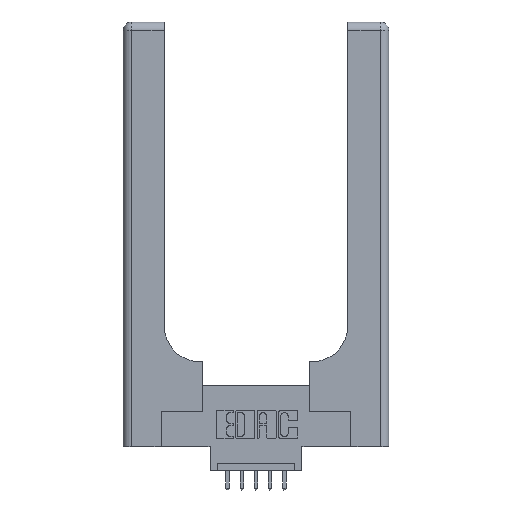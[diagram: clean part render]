
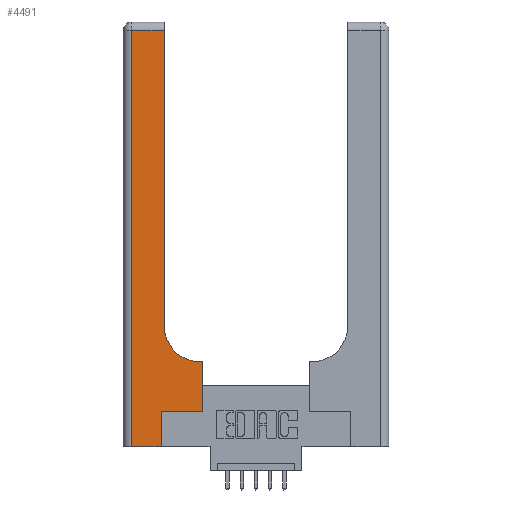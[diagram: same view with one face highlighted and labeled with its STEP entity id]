
A CAD part, top view. The second image highlights one B-rep face of the part: STEP entity #4491.
In plain terms, the highlighted planar face has unit normal (0, 0, 1).
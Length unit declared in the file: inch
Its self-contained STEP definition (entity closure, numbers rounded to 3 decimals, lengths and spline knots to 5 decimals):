
#84 = VERTEX_POINT ( 'NONE', #10954 ) ;
#95 = CARTESIAN_POINT ( 'NONE',  ( 0.5585, 0.6, 0.37 ) ) ;
#163 = CARTESIAN_POINT ( 'NONE',  ( 0., 2.94, 0.37 ) ) ;
#602 = EDGE_CURVE ( 'NONE', #12615, #5786, #12269, .T. ) ;
#630 = VERTEX_POINT ( 'NONE', #1063 ) ;
#729 = CARTESIAN_POINT ( 'NONE',  ( 0.5585, 0.25, 0.37 ) ) ;
#740 = DIRECTION ( 'NONE',  ( -1., 0., 0. ) ) ;
#837 = LINE ( 'NONE', #8546, #9173 ) ;
#874 = LINE ( 'NONE', #163, #2252 ) ;
#981 = EDGE_LOOP ( 'NONE', ( #1285, #3041, #1829, #11075, #13214, #6369, #5208, #11336, #6396 ) ) ;
#1063 = CARTESIAN_POINT ( 'NONE',  ( 0.2915, 2.94, 0.37 ) ) ;
#1086 = EDGE_CURVE ( 'NONE', #630, #84, #874, .T. ) ;
#1156 = LINE ( 'NONE', #11739, #12014 ) ;
#1285 = ORIENTED_EDGE ( 'NONE', *, *, #5250, .T. ) ;
#1527 = CARTESIAN_POINT ( 'NONE',  ( 0.5585, 0.25, 0.37 ) ) ;
#1829 = ORIENTED_EDGE ( 'NONE', *, *, #3646, .T. ) ;
#2144 = LINE ( 'NONE', #4694, #4711 ) ;
#2155 = VECTOR ( 'NONE', #2379, 39.37008 ) ;
#2252 = VECTOR ( 'NONE', #5513, 39.37008 ) ;
#2379 = DIRECTION ( 'NONE',  ( 1., 0., 0. ) ) ;
#2525 = CARTESIAN_POINT ( 'NONE',  ( 0., 0., 0.37 ) ) ;
#2551 = VERTEX_POINT ( 'NONE', #1527 ) ;
#3041 = ORIENTED_EDGE ( 'NONE', *, *, #1086, .T. ) ;
#3265 = DIRECTION ( 'NONE',  ( 0., 1., 0. ) ) ;
#3340 = EDGE_CURVE ( 'NONE', #7024, #4794, #3361, .T. ) ;
#3361 = LINE ( 'NONE', #2525, #2155 ) ;
#3646 = EDGE_CURVE ( 'NONE', #84, #7024, #2144, .T. ) ;
#3764 = VERTEX_POINT ( 'NONE', #95 ) ;
#4142 = CARTESIAN_POINT ( 'NONE',  ( 0.2915, 0.6, 0.37 ) ) ;
#4491 = ADVANCED_FACE ( 'NONE', ( #9932 ), #14074, .F. ) ;
#4560 = CARTESIAN_POINT ( 'NONE',  ( 0.269, 0., 0.37 ) ) ;
#4694 = CARTESIAN_POINT ( 'NONE',  ( 0.06, 3., 0.37 ) ) ;
#4711 = VECTOR ( 'NONE', #10084, 39.37008 ) ;
#4794 = VERTEX_POINT ( 'NONE', #4560 ) ;
#5123 = DIRECTION ( 'NONE',  ( 0., 1., 0. ) ) ;
#5208 = ORIENTED_EDGE ( 'NONE', *, *, #7692, .T. ) ;
#5250 = EDGE_CURVE ( 'NONE', #5786, #630, #7533, .T. ) ;
#5270 = DIRECTION ( 'NONE',  ( 1., 0., 0. ) ) ;
#5277 = CARTESIAN_POINT ( 'NONE',  ( 0.2915, 3., 0.37 ) ) ;
#5471 = LINE ( 'NONE', #729, #13265 ) ;
#5513 = DIRECTION ( 'NONE',  ( -1., 0., 0. ) ) ;
#5786 = VERTEX_POINT ( 'NONE', #6059 ) ;
#6059 = CARTESIAN_POINT ( 'NONE',  ( 0.2915, 0.85, 0.37 ) ) ;
#6262 = LINE ( 'NONE', #4142, #8427 ) ;
#6369 = ORIENTED_EDGE ( 'NONE', *, *, #9356, .T. ) ;
#6396 = ORIENTED_EDGE ( 'NONE', *, *, #602, .T. ) ;
#6500 = CARTESIAN_POINT ( 'NONE',  ( 0.5415, 0.6, 0.37 ) ) ;
#7024 = VERTEX_POINT ( 'NONE', #13681 ) ;
#7426 = DIRECTION ( 'NONE',  ( 0., 0., -1. ) ) ;
#7509 = EDGE_CURVE ( 'NONE', #4794, #9767, #837, .T. ) ;
#7533 = LINE ( 'NONE', #5277, #9581 ) ;
#7692 = EDGE_CURVE ( 'NONE', #2551, #3764, #5471, .T. ) ;
#8357 = DIRECTION ( 'NONE',  ( 0., 0., -1. ) ) ;
#8427 = VECTOR ( 'NONE', #740, 39.37008 ) ;
#8546 = CARTESIAN_POINT ( 'NONE',  ( 0.269, 0., 0.37 ) ) ;
#8560 = DIRECTION ( 'NONE',  ( 0., 1., 0. ) ) ;
#9173 = VECTOR ( 'NONE', #3265, 39.37008 ) ;
#9275 = EDGE_CURVE ( 'NONE', #3764, #12615, #6262, .T. ) ;
#9356 = EDGE_CURVE ( 'NONE', #9767, #2551, #1156, .T. ) ;
#9581 = VECTOR ( 'NONE', #8560, 39.37008 ) ;
#9713 = CARTESIAN_POINT ( 'NONE',  ( 0., 3., 0.37 ) ) ;
#9767 = VERTEX_POINT ( 'NONE', #10281 ) ;
#9932 = FACE_OUTER_BOUND ( 'NONE', #981, .T. ) ;
#10084 = DIRECTION ( 'NONE',  ( 0., -1., 0. ) ) ;
#10281 = CARTESIAN_POINT ( 'NONE',  ( 0.269, 0.25, 0.37 ) ) ;
#10954 = CARTESIAN_POINT ( 'NONE',  ( 0.06, 2.94, 0.37 ) ) ;
#11075 = ORIENTED_EDGE ( 'NONE', *, *, #3340, .T. ) ;
#11336 = ORIENTED_EDGE ( 'NONE', *, *, #9275, .T. ) ;
#11586 = DIRECTION ( 'NONE',  ( 1., 0., 0. ) ) ;
#11739 = CARTESIAN_POINT ( 'NONE',  ( 0.269, 0.25, 0.37 ) ) ;
#12014 = VECTOR ( 'NONE', #5270, 39.37008 ) ;
#12269 = CIRCLE ( 'NONE', #13465, 0.25 ) ;
#12615 = VERTEX_POINT ( 'NONE', #6500 ) ;
#12730 = CARTESIAN_POINT ( 'NONE',  ( 0.5415, 0.85, 0.37 ) ) ;
#13214 = ORIENTED_EDGE ( 'NONE', *, *, #7509, .T. ) ;
#13265 = VECTOR ( 'NONE', #5123, 39.37008 ) ;
#13320 = AXIS2_PLACEMENT_3D ( 'NONE', #9713, #7426, #13889 ) ;
#13465 = AXIS2_PLACEMENT_3D ( 'NONE', #12730, #8357, #11586 ) ;
#13681 = CARTESIAN_POINT ( 'NONE',  ( 0.06, 0., 0.37 ) ) ;
#13889 = DIRECTION ( 'NONE',  ( -1., 0., 0. ) ) ;
#14074 = PLANE ( 'NONE',  #13320 ) ;
